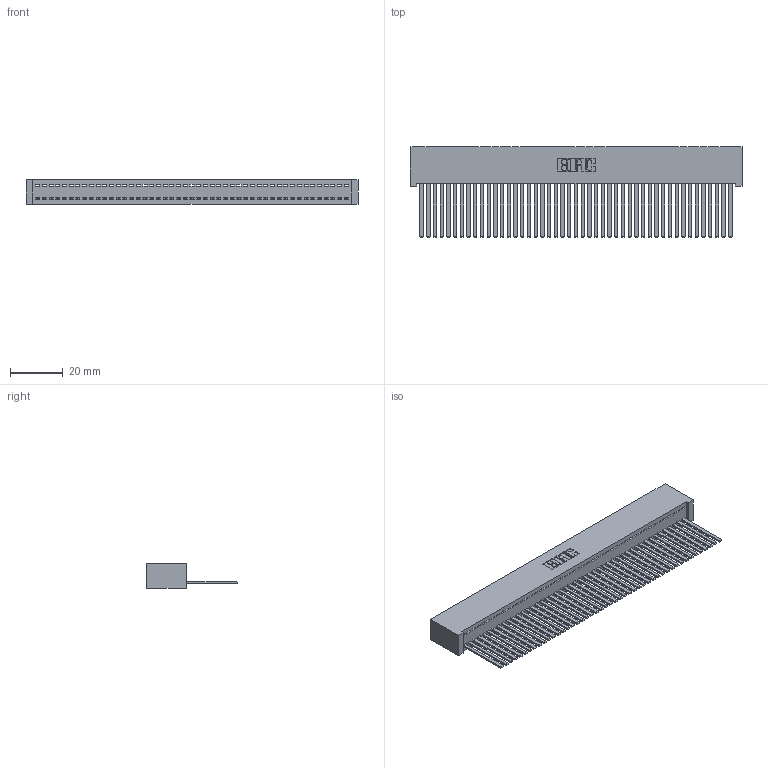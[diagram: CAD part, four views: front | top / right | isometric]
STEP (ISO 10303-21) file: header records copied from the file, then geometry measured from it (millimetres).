
FILE_DESCRIPTION (( 'STEP AP203' ), '1' );
FILE_NAME ('342-047-544-101.STEP', '2019-10-02T21:26:16', ( '' ), ( '' ), 'SwSTEP 2.0', 'SolidWorks 2016', '' );
FILE_SCHEMA (( 'CONFIG_CONTROL_DESIGN' ));
Length unit declared in the file: inch
Products named in the file (3): 342 Part_Lugless; 345-292-001_345-293-144; 342-047-544-101
Assembly tree (48 placements, depth 2):
  342-047-544-101
    342 Part_Lugless
    345-292-001_345-293-144  x47
Bounding box: 125.63 x 34.3 x 9.4 mm (x, y, z)
Volume: 11986.8 mm3; surface area: 19567.9 mm2
Topology: 48 solids, 48 shells, 2546 faces, 7701 edges, 5070 vertices
Faces by surface type: plane 1848, cylinder 698
Entity records: 27493 total; most frequent: CARTESIAN_POINT 4747, ORIENTED_EDGE 4730, DIRECTION 3983, EDGE_CURVE 2365, LINE 2249, VECTOR 2249, VERTEX_POINT 1574, AXIS2_PLACEMENT_3D 867
